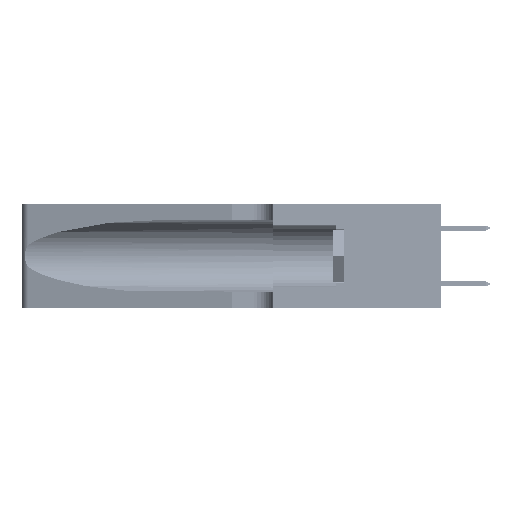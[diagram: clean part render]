
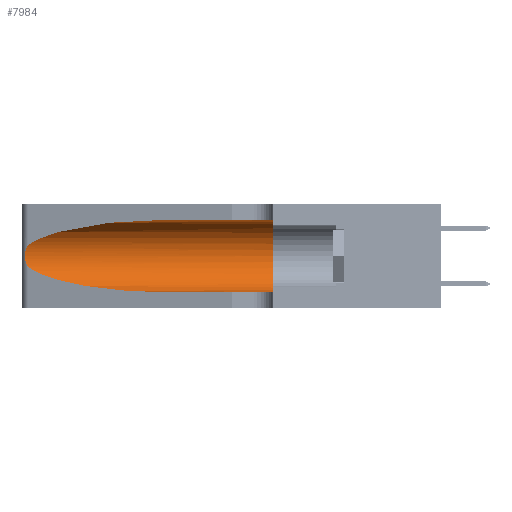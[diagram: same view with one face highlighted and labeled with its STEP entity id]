
A CAD part, left-side view. The second image highlights one B-rep face of the part: STEP entity #7984.
In plain terms, the highlighted cylindrical face has radius 3.308 mm (diameter 6.617 mm), a partial arc.
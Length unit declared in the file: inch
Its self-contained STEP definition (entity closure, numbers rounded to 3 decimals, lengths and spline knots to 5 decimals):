
#46 = EDGE_CURVE ( 'NONE', #13213, #48490, #47182, .T. ) ;
#171 = EDGE_CURVE ( 'NONE', #39556, #10070, #3007, .T. ) ;
#244 = DIRECTION ( 'NONE',  ( 0., -1., 0. ) ) ;
#663 = VERTEX_POINT ( 'NONE', #10926 ) ;
#2606 = EDGE_CURVE ( 'NONE', #13213, #663, #35670, .T. ) ;
#2971 = CARTESIAN_POINT ( 'NONE',  ( 0.25856, 1.23593, 0.16098 ) ) ;
#3007 = LINE ( 'NONE', #43143, #5478 ) ;
#5478 = VECTOR ( 'NONE', #39296, 39.37008 ) ;
#6050 = CARTESIAN_POINT ( 'NONE',  ( 0.1305, 0.72297, 0.31525 ) ) ;
#6752 = CARTESIAN_POINT ( 'NONE',  ( 0.25487, 1.22718, 0.22369 ) ) ;
#6826 = AXIS2_PLACEMENT_3D ( 'NONE', #21814, #48693, #25707 ) ;
#6936 = CARTESIAN_POINT ( 'NONE',  ( 0.25639, 1.23186, 0.15144 ) ) ;
#7560 = CARTESIAN_POINT ( 'NONE',  ( 0.25487, 1.22718, 0.22369 ) ) ;
#7785 = CIRCLE ( 'NONE', #6826, 0.13025 ) ;
#7837 = CARTESIAN_POINT ( 'NONE',  ( 0.1305, 0.72297, 0.05475 ) ) ;
#7984 = ADVANCED_FACE ( 'NONE', ( #32041 ), #11357, .F. ) ;
#8172 = DIRECTION ( 'NONE',  ( 0., 0., -1. ) ) ;
#9054 = AXIS2_PLACEMENT_3D ( 'NONE', #11953, #244, #8172 ) ;
#10070 = VERTEX_POINT ( 'NONE', #47579 ) ;
#10873 = CARTESIAN_POINT ( 'NONE',  ( 0.25487, 1.22718, 0.14631 ) ) ;
#10926 = CARTESIAN_POINT ( 'NONE',  ( 0.1305, 0.35, 0.31525 ) ) ;
#11357 = CYLINDRICAL_SURFACE ( 'NONE', #9054, 0.13025 ) ;
#11953 = CARTESIAN_POINT ( 'NONE',  ( 0.1305, 1.61858, 0.185 ) ) ;
#12779 = B_SPLINE_CURVE_WITH_KNOTS ( 'NONE', 3,
 ( #6752, #18454, #14648, #41700, #18622, #45554, #22512, #49372, #26400, #2971, #30274, #6936, #34142, #10873 ),
 .UNSPECIFIED., .F., .F.,
 ( 4, 2, 2, 2, 2, 2, 4 ),
 ( 0., 0.00027, 0.00053, 0.00107, 0.0016, 0.00187, 0.00214 ),
 .UNSPECIFIED. ) ;
#13213 = VERTEX_POINT ( 'NONE', #6050 ) ;
#14557 = ORIENTED_EDGE ( 'NONE', *, *, #43549, .T. ) ;
#14648 = CARTESIAN_POINT ( 'NONE',  ( 0.25639, 1.23184, 0.21858 ) ) ;
#15031 = VECTOR ( 'NONE', #26548, 39.37008 ) ;
#16474 = CARTESIAN_POINT ( 'NONE',  ( 0.25487, 1.22718, 0.14631 ) ) ;
#18454 = CARTESIAN_POINT ( 'NONE',  ( 0.25555, 1.22994, 0.2215 ) ) ;
#18622 = CARTESIAN_POINT ( 'NONE',  ( 0.25854, 1.2359, 0.20912 ) ) ;
#19731 = VERTEX_POINT ( 'NONE', #44988 ) ;
#20924 = EDGE_CURVE ( 'NONE', #48490, #19731, #12779, .T. ) ;
#21814 = CARTESIAN_POINT ( 'NONE',  ( 0.1305, 0.35, 0.185 ) ) ;
#22512 = CARTESIAN_POINT ( 'NONE',  ( 0.26075, 1.23896, 0.19203 ) ) ;
#23137 = CARTESIAN_POINT ( 'NONE',  ( 0.18966, 0.96281, 0.31525 ) ) ;
#23318 = EDGE_LOOP ( 'NONE', ( #42440, #32781, #14557, #30076, #32399, #45484 ) ) ;
#24286 = CARTESIAN_POINT ( 'NONE',  ( 0.1305, 0.72297, 0.05475 ) ) ;
#25707 = DIRECTION ( 'NONE',  ( 0., 0., 1. ) ) ;
#26400 = CARTESIAN_POINT ( 'NONE',  ( 0.26017, 1.23833, 0.17102 ) ) ;
#26548 = DIRECTION ( 'NONE',  ( 0., -1., 0. ) ) ;
#30076 = ORIENTED_EDGE ( 'NONE', *, *, #171, .T. ) ;
#30274 = CARTESIAN_POINT ( 'NONE',  ( 0.25789, 1.23486, 0.15765 ) ) ;
#30893 = CARTESIAN_POINT ( 'NONE',  ( 0.1305, 0.72297, 0.31525 ) ) ;
#32041 = FACE_OUTER_BOUND ( 'NONE', #23318, .T. ) ;
#32399 = ORIENTED_EDGE ( 'NONE', *, *, #33753, .F. ) ;
#32781 = ORIENTED_EDGE ( 'NONE', *, *, #20924, .T. ) ;
#33753 = EDGE_CURVE ( 'NONE', #663, #10070, #7785, .T. ) ;
#34142 = CARTESIAN_POINT ( 'NONE',  ( 0.25555, 1.22993, 0.14849 ) ) ;
#35670 = LINE ( 'NONE', #49531, #15031 ) ;
#35800 =( BOUNDED_CURVE ( )  B_SPLINE_CURVE ( 3, ( #16474, #39618, #47316, #24286 ),
 .UNSPECIFIED., .F., .F. ) 
 B_SPLINE_CURVE_WITH_KNOTS ( ( 4, 4 ),
 ( 3.44316, 4.71239 ),
 .UNSPECIFIED. ) 
 CURVE ( )  GEOMETRIC_REPRESENTATION_ITEM ( )  RATIONAL_B_SPLINE_CURVE ( ( 1., 0.87, 0.87, 1. ) ) 
 REPRESENTATION_ITEM ( '' )  );
#39296 = DIRECTION ( 'NONE',  ( 0., -1., 0. ) ) ;
#39556 = VERTEX_POINT ( 'NONE', #7837 ) ;
#39618 = CARTESIAN_POINT ( 'NONE',  ( 0.2373, 1.15595, 0.08982 ) ) ;
#41495 = CARTESIAN_POINT ( 'NONE',  ( 0.25487, 1.22718, 0.22369 ) ) ;
#41700 = CARTESIAN_POINT ( 'NONE',  ( 0.25787, 1.23484, 0.2124 ) ) ;
#42440 = ORIENTED_EDGE ( 'NONE', *, *, #46, .T. ) ;
#43143 = CARTESIAN_POINT ( 'NONE',  ( 0.1305, 1.61858, 0.05475 ) ) ;
#43549 = EDGE_CURVE ( 'NONE', #19731, #39556, #35800, .T. ) ;
#44988 = CARTESIAN_POINT ( 'NONE',  ( 0.25487, 1.22718, 0.14631 ) ) ;
#45484 = ORIENTED_EDGE ( 'NONE', *, *, #2606, .F. ) ;
#45554 = CARTESIAN_POINT ( 'NONE',  ( 0.26018, 1.23835, 0.19895 ) ) ;
#46168 = CARTESIAN_POINT ( 'NONE',  ( 0.2373, 1.15595, 0.28018 ) ) ;
#47182 =( BOUNDED_CURVE ( )  B_SPLINE_CURVE ( 3, ( #30893, #23137, #46168, #7560 ),
 .UNSPECIFIED., .F., .T. ) 
 B_SPLINE_CURVE_WITH_KNOTS ( ( 4, 4 ),
 ( 1.5708, 2.84003 ),
 .UNSPECIFIED. ) 
 CURVE ( )  GEOMETRIC_REPRESENTATION_ITEM ( )  RATIONAL_B_SPLINE_CURVE ( ( 1., 0.87, 0.87, 1. ) ) 
 REPRESENTATION_ITEM ( '' )  );
#47316 = CARTESIAN_POINT ( 'NONE',  ( 0.18966, 0.96281, 0.05475 ) ) ;
#47579 = CARTESIAN_POINT ( 'NONE',  ( 0.1305, 0.35, 0.05475 ) ) ;
#48490 = VERTEX_POINT ( 'NONE', #41495 ) ;
#48693 = DIRECTION ( 'NONE',  ( 0., 1., 0. ) ) ;
#49372 = CARTESIAN_POINT ( 'NONE',  ( 0.26075, 1.23896, 0.178 ) ) ;
#49531 = CARTESIAN_POINT ( 'NONE',  ( 0.1305, 1.61858, 0.31525 ) ) ;
